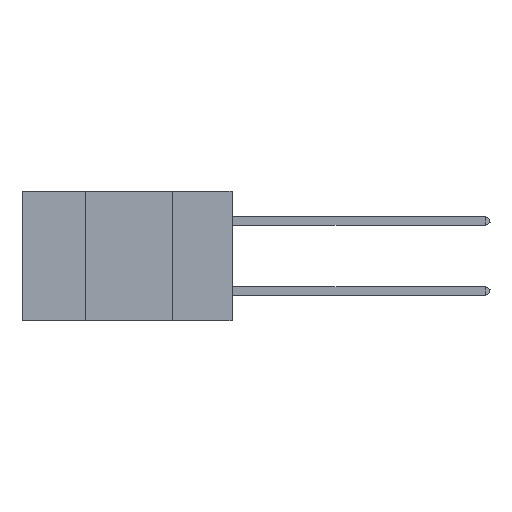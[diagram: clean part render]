
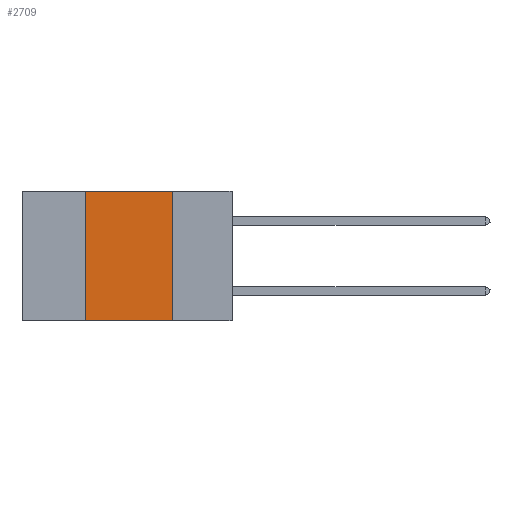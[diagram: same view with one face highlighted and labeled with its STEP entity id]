
A CAD part, left-side view. The second image highlights one B-rep face of the part: STEP entity #2709.
In plain terms, the highlighted planar face has unit normal (-1, 0, 0).
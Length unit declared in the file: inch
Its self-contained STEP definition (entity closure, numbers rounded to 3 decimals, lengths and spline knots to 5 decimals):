
#1055 = DIRECTION ( 'NONE',  ( 1., 0., 0. ) ) ;
#2709 = ADVANCED_FACE ( 'NONE', ( #3327 ), #6091, .F. ) ;
#3327 = FACE_OUTER_BOUND ( 'NONE', #30873, .T. ) ;
#3552 = AXIS2_PLACEMENT_3D ( 'NONE', #6663, #1055, #18326 ) ;
#4286 = DIRECTION ( 'NONE',  ( 0., 0., -1. ) ) ;
#5627 = EDGE_CURVE ( 'NONE', #9962, #9434, #11594, .T. ) ;
#6091 = PLANE ( 'NONE',  #3552 ) ;
#6663 = CARTESIAN_POINT ( 'NONE',  ( 0., 0.6, 0. ) ) ;
#8189 = DIRECTION ( 'NONE',  ( 0., 0., 1. ) ) ;
#9434 = VERTEX_POINT ( 'NONE', #16006 ) ;
#9581 = CARTESIAN_POINT ( 'NONE',  ( 0., 0.42, -0.37 ) ) ;
#9890 = ORIENTED_EDGE ( 'NONE', *, *, #13270, .T. ) ;
#9962 = VERTEX_POINT ( 'NONE', #9581 ) ;
#10132 = LINE ( 'NONE', #16264, #16857 ) ;
#10325 = LINE ( 'NONE', #21491, #17964 ) ;
#11594 = LINE ( 'NONE', #27391, #33417 ) ;
#13270 = EDGE_CURVE ( 'NONE', #9962, #33554, #10325, .T. ) ;
#16006 = CARTESIAN_POINT ( 'NONE',  ( 0., 0.42, 0. ) ) ;
#16264 = CARTESIAN_POINT ( 'NONE',  ( 0., 0.6, 0. ) ) ;
#16819 = ORIENTED_EDGE ( 'NONE', *, *, #26641, .F. ) ;
#16857 = VECTOR ( 'NONE', #19159, 39.37008 ) ;
#17568 = EDGE_CURVE ( 'NONE', #9434, #18476, #10132, .T. ) ;
#17964 = VECTOR ( 'NONE', #35571, 39.37008 ) ;
#18326 = DIRECTION ( 'NONE',  ( 0., 0., -1. ) ) ;
#18476 = VERTEX_POINT ( 'NONE', #34965 ) ;
#19159 = DIRECTION ( 'NONE',  ( 0., -1., 0. ) ) ;
#21390 = CARTESIAN_POINT ( 'NONE',  ( 0., 0.17, 0. ) ) ;
#21491 = CARTESIAN_POINT ( 'NONE',  ( 0., 0.6, -0.37 ) ) ;
#22576 = LINE ( 'NONE', #21390, #23488 ) ;
#23488 = VECTOR ( 'NONE', #4286, 39.37008 ) ;
#26641 = EDGE_CURVE ( 'NONE', #18476, #33554, #22576, .T. ) ;
#27391 = CARTESIAN_POINT ( 'NONE',  ( 0., 0.42, 0. ) ) ;
#27475 = ORIENTED_EDGE ( 'NONE', *, *, #5627, .F. ) ;
#28901 = CARTESIAN_POINT ( 'NONE',  ( 0., 0.17, -0.37 ) ) ;
#30873 = EDGE_LOOP ( 'NONE', ( #16819, #33090, #27475, #9890 ) ) ;
#33090 = ORIENTED_EDGE ( 'NONE', *, *, #17568, .F. ) ;
#33417 = VECTOR ( 'NONE', #8189, 39.37008 ) ;
#33554 = VERTEX_POINT ( 'NONE', #28901 ) ;
#34965 = CARTESIAN_POINT ( 'NONE',  ( 0., 0.17, 0. ) ) ;
#35571 = DIRECTION ( 'NONE',  ( 0., -1., 0. ) ) ;
